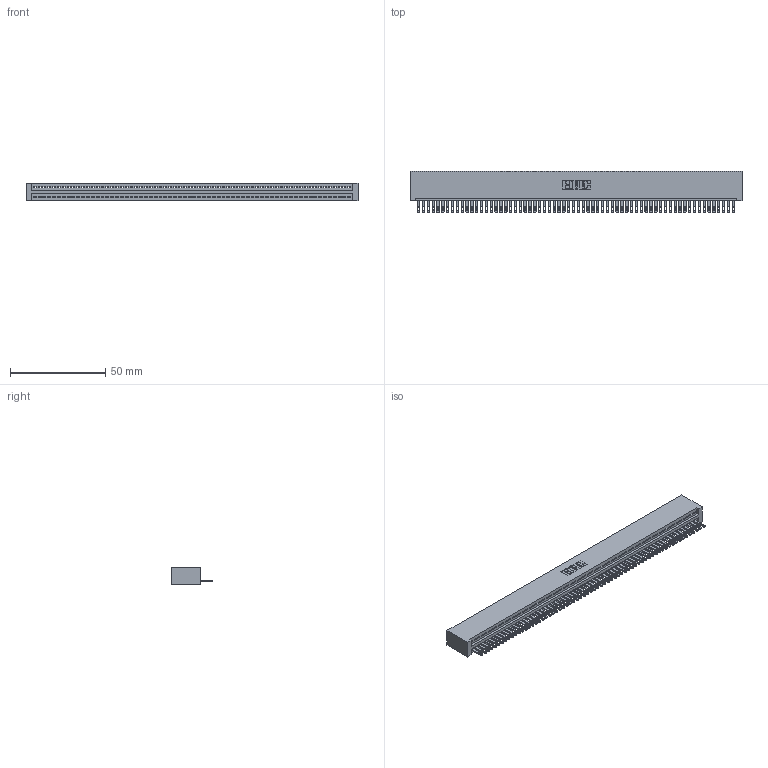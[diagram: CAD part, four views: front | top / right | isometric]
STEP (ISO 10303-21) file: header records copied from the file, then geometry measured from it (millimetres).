
FILE_DESCRIPTION (( 'STEP AP203' ), '1' );
FILE_NAME ('895-066-500-101.STEP', '2020-09-28T11:59:57', ( '' ), ( '' ), 'SwSTEP 2.0', 'SolidWorks 2020', '' );
FILE_SCHEMA (( 'CONFIG_CONTROL_DESIGN' ));
Length unit declared in the file: inch
Products named in the file (3): 345-292-001_345-293-100; 895-066-500-101; 845 Part_No Mounting Lugs
Assembly tree (67 placements, depth 2):
  895-066-500-101
    845 Part_No Mounting Lugs
    345-292-001_345-293-100  x66
Bounding box: 174.24 x 21.51 x 9.4 mm (x, y, z)
Volume: 17371.7 mm3; surface area: 23749.9 mm2
Topology: 67 solids, 67 shells, 3682 faces, 11405 edges, 7602 vertices
Faces by surface type: plane 2320, cylinder 1362
Entity records: 46095 total; most frequent: CARTESIAN_POINT 7990, ORIENTED_EDGE 7990, DIRECTION 6939, EDGE_CURVE 3995, LINE 3603, VECTOR 3603, VERTEX_POINT 2662, AXIS2_PLACEMENT_3D 1668
